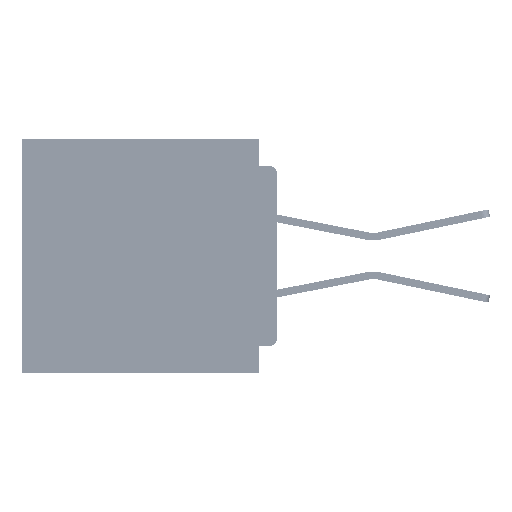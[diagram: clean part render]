
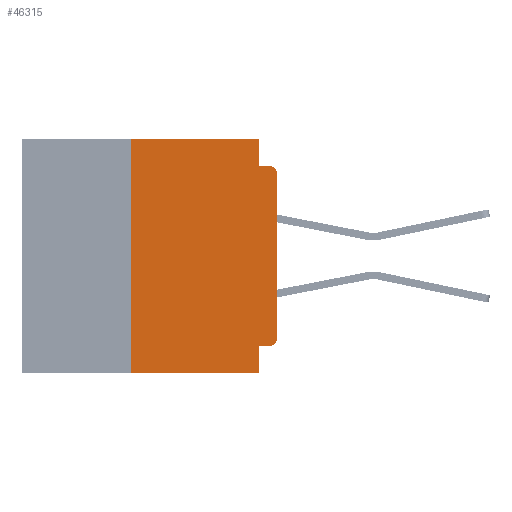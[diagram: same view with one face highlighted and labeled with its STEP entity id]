
A CAD part, left-side view. The second image highlights one B-rep face of the part: STEP entity #46315.
In plain terms, the highlighted planar face has unit normal (-1, 0, 0).
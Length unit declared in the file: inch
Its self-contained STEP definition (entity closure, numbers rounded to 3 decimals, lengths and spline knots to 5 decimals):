
#1419 = VECTOR ( 'NONE', #21100, 39.37008 ) ;
#2608 = DIRECTION ( 'NONE',  ( 0., 0., -1. ) ) ;
#4522 = CARTESIAN_POINT ( 'NONE',  ( 0., 0., -0.06 ) ) ;
#5791 = CARTESIAN_POINT ( 'NONE',  ( 0., 0.437, 0. ) ) ;
#6131 = EDGE_CURVE ( 'NONE', #52779, #52347, #53966, .T. ) ;
#7733 = ORIENTED_EDGE ( 'NONE', *, *, #22450, .F. ) ;
#9376 = CARTESIAN_POINT ( 'NONE',  ( 0., 0., -0.34 ) ) ;
#9452 = LINE ( 'NONE', #31318, #63852 ) ;
#10101 = EDGE_LOOP ( 'NONE', ( #50171, #12196, #27542, #61644, #38366, #28572, #61400, #7733, #52891, #42249 ) ) ;
#11161 = DIRECTION ( 'NONE',  ( 0., 0., -1. ) ) ;
#12196 = ORIENTED_EDGE ( 'NONE', *, *, #21023, .T. ) ;
#13428 = EDGE_CURVE ( 'NONE', #25160, #16160, #17533, .T. ) ;
#13855 = CARTESIAN_POINT ( 'NONE',  ( 0., 0.015, -0.34 ) ) ;
#16160 = VERTEX_POINT ( 'NONE', #35069 ) ;
#16548 = LINE ( 'NONE', #26967, #27334 ) ;
#17215 = LINE ( 'NONE', #47362, #1419 ) ;
#17533 = LINE ( 'NONE', #31007, #20876 ) ;
#18899 = VECTOR ( 'NONE', #31309, 39.37008 ) ;
#19229 = DIRECTION ( 'NONE',  ( 0., 0., -1. ) ) ;
#20600 = AXIS2_PLACEMENT_3D ( 'NONE', #13855, #50780, #19229 ) ;
#20876 = VECTOR ( 'NONE', #67664, 39.37008 ) ;
#21023 = EDGE_CURVE ( 'NONE', #59307, #46352, #45037, .T. ) ;
#21100 = DIRECTION ( 'NONE',  ( 0., 0., -1. ) ) ;
#22395 = EDGE_CURVE ( 'NONE', #52347, #38609, #32970, .T. ) ;
#22450 = EDGE_CURVE ( 'NONE', #36091, #16160, #17215, .T. ) ;
#25160 = VERTEX_POINT ( 'NONE', #36237 ) ;
#25188 = CARTESIAN_POINT ( 'NONE',  ( 0., 0., 0. ) ) ;
#26967 = CARTESIAN_POINT ( 'NONE',  ( 0., 0., -0.045 ) ) ;
#27334 = VECTOR ( 'NONE', #58624, 39.37008 ) ;
#27542 = ORIENTED_EDGE ( 'NONE', *, *, #53694, .F. ) ;
#27545 = VECTOR ( 'NONE', #35561, 39.37008 ) ;
#28572 = ORIENTED_EDGE ( 'NONE', *, *, #42863, .F. ) ;
#30890 = AXIS2_PLACEMENT_3D ( 'NONE', #65751, #34391, #2608 ) ;
#31007 = CARTESIAN_POINT ( 'NONE',  ( 0., 0.437, -0.4 ) ) ;
#31309 = DIRECTION ( 'NONE',  ( 0., 0., -1. ) ) ;
#31318 = CARTESIAN_POINT ( 'NONE',  ( 0., 0., -0.355 ) ) ;
#32970 = LINE ( 'NONE', #41616, #18899 ) ;
#33551 = CARTESIAN_POINT ( 'NONE',  ( 0., 0.25, 0. ) ) ;
#34391 = DIRECTION ( 'NONE',  ( -1., 0., 0. ) ) ;
#35069 = CARTESIAN_POINT ( 'NONE',  ( 0., 0.031, -0.4 ) ) ;
#35456 = DIRECTION ( 'NONE',  ( 0., -1., 0. ) ) ;
#35561 = DIRECTION ( 'NONE',  ( 0., 0., 1. ) ) ;
#36091 = VERTEX_POINT ( 'NONE', #51373 ) ;
#36237 = CARTESIAN_POINT ( 'NONE',  ( 0., 0.25, -0.4 ) ) ;
#37286 = CIRCLE ( 'NONE', #20600, 0.015 ) ;
#38366 = ORIENTED_EDGE ( 'NONE', *, *, #6131, .F. ) ;
#38609 = VERTEX_POINT ( 'NONE', #46708 ) ;
#41550 = VECTOR ( 'NONE', #65760, 39.37008 ) ;
#41616 = CARTESIAN_POINT ( 'NONE',  ( 0., 0.031, 0. ) ) ;
#41828 = EDGE_CURVE ( 'NONE', #65714, #36091, #9452, .T. ) ;
#42249 = ORIENTED_EDGE ( 'NONE', *, *, #65629, .T. ) ;
#42824 = DIRECTION ( 'NONE',  ( 1., 0., 0. ) ) ;
#42863 = EDGE_CURVE ( 'NONE', #25160, #52779, #57162, .T. ) ;
#43616 = FACE_OUTER_BOUND ( 'NONE', #10101, .T. ) ;
#45037 = CIRCLE ( 'NONE', #30890, 0.015 ) ;
#46315 = ADVANCED_FACE ( 'NONE', ( #43616 ), #58394, .F. ) ;
#46352 = VERTEX_POINT ( 'NONE', #53358 ) ;
#46708 = CARTESIAN_POINT ( 'NONE',  ( 0., 0.031, -0.045 ) ) ;
#47362 = CARTESIAN_POINT ( 'NONE',  ( 0., 0.031, -0.4 ) ) ;
#50171 = ORIENTED_EDGE ( 'NONE', *, *, #58568, .T. ) ;
#50671 = VECTOR ( 'NONE', #35456, 39.37008 ) ;
#50780 = DIRECTION ( 'NONE',  ( -1., 0., 0. ) ) ;
#51043 = CARTESIAN_POINT ( 'NONE',  ( 0., 0.437, 0. ) ) ;
#51373 = CARTESIAN_POINT ( 'NONE',  ( 0., 0.031, -0.355 ) ) ;
#52012 = AXIS2_PLACEMENT_3D ( 'NONE', #5791, #42824, #11161 ) ;
#52347 = VERTEX_POINT ( 'NONE', #66584 ) ;
#52779 = VERTEX_POINT ( 'NONE', #33551 ) ;
#52891 = ORIENTED_EDGE ( 'NONE', *, *, #41828, .F. ) ;
#53358 = CARTESIAN_POINT ( 'NONE',  ( 0., 0.015, -0.045 ) ) ;
#53694 = EDGE_CURVE ( 'NONE', #38609, #46352, #16548, .T. ) ;
#53966 = LINE ( 'NONE', #51043, #50671 ) ;
#56511 = CARTESIAN_POINT ( 'NONE',  ( 0., 0.015, -0.355 ) ) ;
#57162 = LINE ( 'NONE', #60522, #41550 ) ;
#58394 = PLANE ( 'NONE',  #52012 ) ;
#58568 = EDGE_CURVE ( 'NONE', #66360, #59307, #67769, .T. ) ;
#58624 = DIRECTION ( 'NONE',  ( 0., -1., 0. ) ) ;
#59307 = VERTEX_POINT ( 'NONE', #4522 ) ;
#60522 = CARTESIAN_POINT ( 'NONE',  ( 0., 0.25, -0.4 ) ) ;
#61400 = ORIENTED_EDGE ( 'NONE', *, *, #13428, .T. ) ;
#61644 = ORIENTED_EDGE ( 'NONE', *, *, #22395, .F. ) ;
#63852 = VECTOR ( 'NONE', #67988, 39.37008 ) ;
#65629 = EDGE_CURVE ( 'NONE', #65714, #66360, #37286, .T. ) ;
#65714 = VERTEX_POINT ( 'NONE', #56511 ) ;
#65751 = CARTESIAN_POINT ( 'NONE',  ( 0., 0.015, -0.06 ) ) ;
#65760 = DIRECTION ( 'NONE',  ( 0., 0., 1. ) ) ;
#66360 = VERTEX_POINT ( 'NONE', #9376 ) ;
#66584 = CARTESIAN_POINT ( 'NONE',  ( 0., 0.031, 0. ) ) ;
#67664 = DIRECTION ( 'NONE',  ( 0., -1., 0. ) ) ;
#67769 = LINE ( 'NONE', #25188, #27545 ) ;
#67988 = DIRECTION ( 'NONE',  ( 0., 1., 0. ) ) ;
